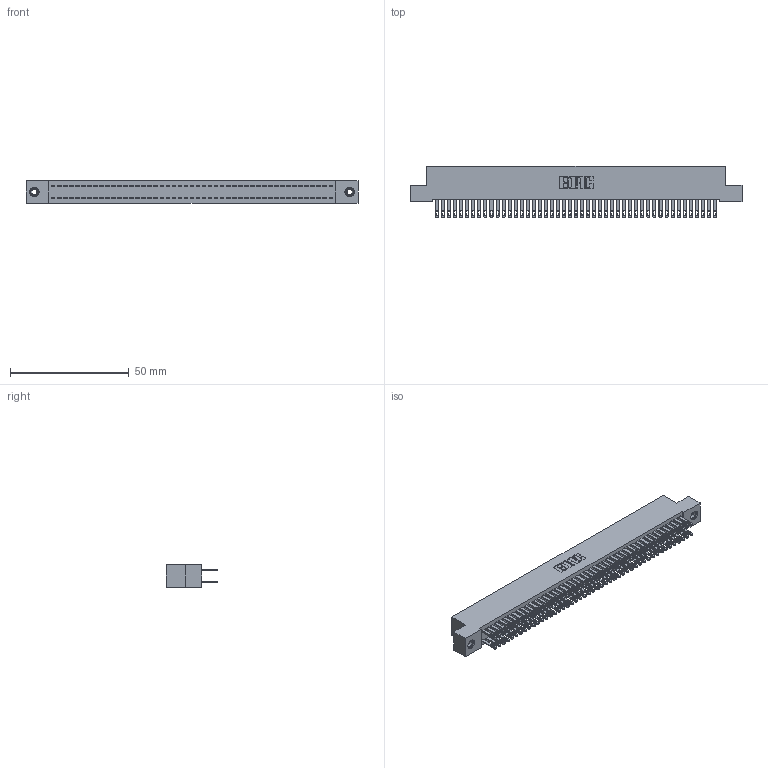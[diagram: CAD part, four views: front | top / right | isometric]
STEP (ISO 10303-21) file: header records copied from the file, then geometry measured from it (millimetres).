
FILE_DESCRIPTION (( 'STEP AP203' ), '1' );
FILE_NAME ('892-094-500-208.STEP', '2020-09-21T21:00:24', ( '' ), ( '' ), 'SwSTEP 2.0', 'SolidWorks 2020', '' );
FILE_SCHEMA (( 'CONFIG_CONTROL_DESIGN' ));
Length unit declared in the file: inch
Products named in the file (4): 892-094-500-208; 842 Part_TI; 345-292-001_345-293-100; 345-250-001_345-250-003-102
Assembly tree (97 placements, depth 2):
  892-094-500-208
    842 Part_TI
    345-292-001_345-293-100  x94
    345-250-001_345-250-003-102  x2
Bounding box: 139.7 x 21.85 x 9.4 mm (x, y, z)
Volume: 12857.3 mm3; surface area: 21961.9 mm2
Topology: 97 solids, 97 shells, 4682 faces, 14253 edges, 9494 vertices
Faces by surface type: plane 2918, cylinder 1748, cone 12, torus 4
Entity records: 30574 total; most frequent: CARTESIAN_POINT 5041, ORIENTED_EDGE 4970, DIRECTION 4331, EDGE_CURVE 2485, VECTOR 2333, LINE 2333, VERTEX_POINT 1652, AXIS2_PLACEMENT_3D 999
